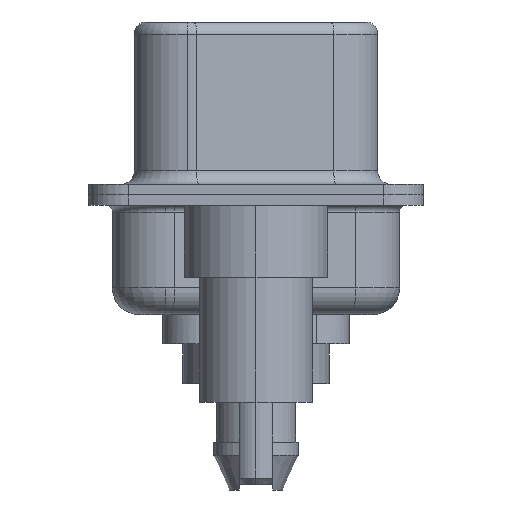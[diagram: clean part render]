
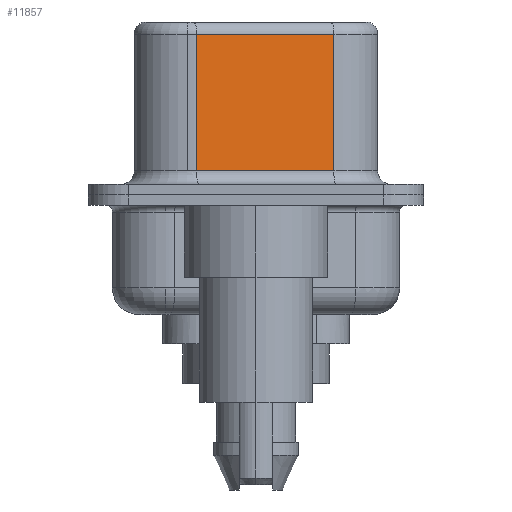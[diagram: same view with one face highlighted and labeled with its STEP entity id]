
A CAD part, left-side view. The second image highlights one B-rep face of the part: STEP entity #11857.
In plain terms, the highlighted planar face has unit normal (-0.985, -0.174, 0).
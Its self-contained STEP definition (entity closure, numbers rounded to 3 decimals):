
#44 = VECTOR ( 'NONE', #14166, 1000. ) ;
#376 = LINE ( 'NONE', #5577, #6252 ) ;
#399 = EDGE_LOOP ( 'NONE', ( #14599, #3746, #10209, #4769 ) ) ;
#441 = VERTEX_POINT ( 'NONE', #6466 ) ;
#785 = CARTESIAN_POINT ( 'NONE',  ( 3.675, 2.233, 0.9 ) ) ;
#1049 = LINE ( 'NONE', #10552, #7687 ) ;
#3746 = ORIENTED_EDGE ( 'NONE', *, *, #9788, .T. ) ;
#4143 = VERTEX_POINT ( 'NONE', #785 ) ;
#4159 = DIRECTION ( 'NONE',  ( 0., 0., -1. ) ) ;
#4473 = CARTESIAN_POINT ( 'NONE',  ( 4.585, -2.927, 6.52 ) ) ;
#4732 = FACE_OUTER_BOUND ( 'NONE', #399, .T. ) ;
#4769 = ORIENTED_EDGE ( 'NONE', *, *, #11289, .T. ) ;
#5544 = EDGE_CURVE ( 'NONE', #11621, #4143, #1049, .T. ) ;
#5577 = CARTESIAN_POINT ( 'NONE',  ( 4.585, -2.927, 6.52 ) ) ;
#5657 = DIRECTION ( 'NONE',  ( -0.174, 0.985, 0. ) ) ;
#6252 = VECTOR ( 'NONE', #6764, 1000. ) ;
#6466 = CARTESIAN_POINT ( 'NONE',  ( 4.585, -2.927, 6.02 ) ) ;
#6491 = VERTEX_POINT ( 'NONE', #9864 ) ;
#6504 = CARTESIAN_POINT ( 'NONE',  ( 3.675, 2.233, 6.02 ) ) ;
#6764 = DIRECTION ( 'NONE',  ( 0., 0., -1. ) ) ;
#6946 = DIRECTION ( 'NONE',  ( 0.174, -0.985, 0. ) ) ;
#7687 = VECTOR ( 'NONE', #4159, 1000. ) ;
#9248 = PLANE ( 'NONE',  #10862 ) ;
#9788 = EDGE_CURVE ( 'NONE', #441, #11621, #9871, .T. ) ;
#9864 = CARTESIAN_POINT ( 'NONE',  ( 4.585, -2.927, 0.9 ) ) ;
#9871 = LINE ( 'NONE', #13038, #44 ) ;
#10209 = ORIENTED_EDGE ( 'NONE', *, *, #5544, .T. ) ;
#10552 = CARTESIAN_POINT ( 'NONE',  ( 3.675, 2.233, 6.52 ) ) ;
#10862 = AXIS2_PLACEMENT_3D ( 'NONE', #4473, #12821, #5657 ) ;
#11228 = EDGE_CURVE ( 'NONE', #441, #6491, #376, .T. ) ;
#11289 = EDGE_CURVE ( 'NONE', #4143, #6491, #11580, .T. ) ;
#11580 = LINE ( 'NONE', #12929, #14988 ) ;
#11621 = VERTEX_POINT ( 'NONE', #6504 ) ;
#11857 = ADVANCED_FACE ( 'NONE', ( #4732 ), #9248, .F. ) ;
#12821 = DIRECTION ( 'NONE',  ( 0.985, 0.174, 0. ) ) ;
#12929 = CARTESIAN_POINT ( 'NONE',  ( 4.585, -2.927, 0.9 ) ) ;
#13038 = CARTESIAN_POINT ( 'NONE',  ( 4.585, -2.927, 6.02 ) ) ;
#14166 = DIRECTION ( 'NONE',  ( -0.174, 0.985, 0. ) ) ;
#14599 = ORIENTED_EDGE ( 'NONE', *, *, #11228, .F. ) ;
#14988 = VECTOR ( 'NONE', #6946, 1000. ) ;
